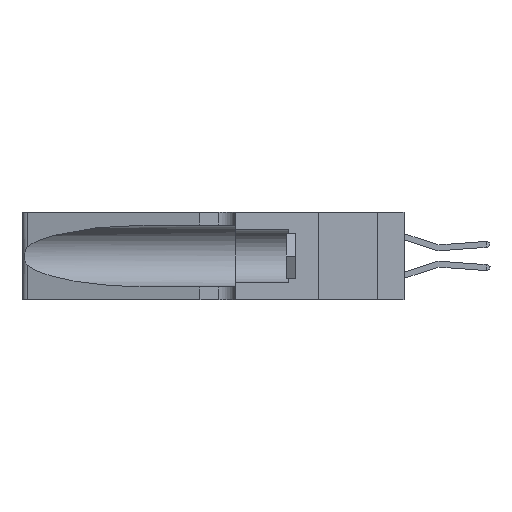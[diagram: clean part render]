
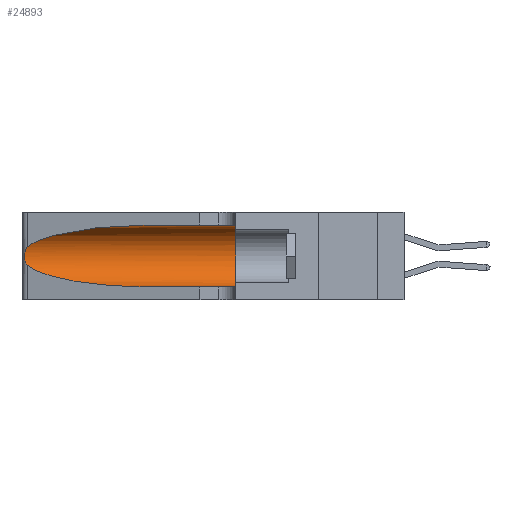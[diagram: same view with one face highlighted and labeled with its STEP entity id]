
A CAD part, left-side view. The second image highlights one B-rep face of the part: STEP entity #24893.
In plain terms, the highlighted cylindrical face has radius 3.308 mm (diameter 6.617 mm), a partial arc.
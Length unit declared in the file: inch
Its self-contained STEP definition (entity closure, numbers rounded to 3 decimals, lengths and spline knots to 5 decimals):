
#464 = CARTESIAN_POINT ( 'NONE',  ( 0.1305, 1.61858, 0.31525 ) ) ;
#783 = CIRCLE ( 'NONE', #27020, 0.13025 ) ;
#978 = CARTESIAN_POINT ( 'NONE',  ( 0.1305, 0.72297, 0.31525 ) ) ;
#1686 = CARTESIAN_POINT ( 'NONE',  ( 0.25487, 1.22718, 0.14631 ) ) ;
#2050 = EDGE_CURVE ( 'NONE', #2422, #31044, #10389, .T. ) ;
#2157 = DIRECTION ( 'NONE',  ( 0., -1., 0. ) ) ;
#2422 = VERTEX_POINT ( 'NONE', #22858 ) ;
#2440 = CARTESIAN_POINT ( 'NONE',  ( 0.1305, 0.35, 0.05475 ) ) ;
#3281 =( BOUNDED_CURVE ( )  B_SPLINE_CURVE ( 3, ( #1686, #19780, #32725, #7276 ),
 .UNSPECIFIED., .F., .F. ) 
 B_SPLINE_CURVE_WITH_KNOTS ( ( 4, 4 ),
 ( 3.44316, 4.71239 ),
 .UNSPECIFIED. ) 
 CURVE ( )  GEOMETRIC_REPRESENTATION_ITEM ( )  RATIONAL_B_SPLINE_CURVE ( ( 1., 0.87, 0.87, 1. ) ) 
 REPRESENTATION_ITEM ( '' )  );
#3384 = CARTESIAN_POINT ( 'NONE',  ( 0.18966, 0.96281, 0.31525 ) ) ;
#4279 = EDGE_CURVE ( 'NONE', #29355, #11122, #783, .T. ) ;
#4359 = VECTOR ( 'NONE', #30156, 39.37008 ) ;
#4670 = CARTESIAN_POINT ( 'NONE',  ( 0.26017, 1.23833, 0.17102 ) ) ;
#5508 = CARTESIAN_POINT ( 'NONE',  ( 0.25856, 1.23593, 0.16098 ) ) ;
#5982 = CARTESIAN_POINT ( 'NONE',  ( 0.2373, 1.15595, 0.28018 ) ) ;
#6266 = LINE ( 'NONE', #9989, #19621 ) ;
#6435 = CARTESIAN_POINT ( 'NONE',  ( 0.25787, 1.23484, 0.2124 ) ) ;
#6599 = ORIENTED_EDGE ( 'NONE', *, *, #18024, .T. ) ;
#7276 = CARTESIAN_POINT ( 'NONE',  ( 0.1305, 0.72297, 0.05475 ) ) ;
#9112 = CARTESIAN_POINT ( 'NONE',  ( 0.25555, 1.22993, 0.14849 ) ) ;
#9121 = EDGE_LOOP ( 'NONE', ( #25221, #6599, #23235, #28453, #20481, #32669 ) ) ;
#9911 = DIRECTION ( 'NONE',  ( 0., 1., 0. ) ) ;
#9989 = CARTESIAN_POINT ( 'NONE',  ( 0.1305, 1.61858, 0.05475 ) ) ;
#10095 = EDGE_CURVE ( 'NONE', #12147, #11122, #6266, .T. ) ;
#10389 =( BOUNDED_CURVE ( )  B_SPLINE_CURVE ( 3, ( #978, #3384, #5982, #32279 ),
 .UNSPECIFIED., .F., .F. ) 
 B_SPLINE_CURVE_WITH_KNOTS ( ( 4, 4 ),
 ( 1.5708, 2.84003 ),
 .UNSPECIFIED. ) 
 CURVE ( )  GEOMETRIC_REPRESENTATION_ITEM ( )  RATIONAL_B_SPLINE_CURVE ( ( 1., 0.87, 0.87, 1. ) ) 
 REPRESENTATION_ITEM ( '' )  );
#10783 = CARTESIAN_POINT ( 'NONE',  ( 0.25639, 1.23184, 0.21858 ) ) ;
#11122 = VERTEX_POINT ( 'NONE', #2440 ) ;
#11601 = CARTESIAN_POINT ( 'NONE',  ( 0.25639, 1.23186, 0.15144 ) ) ;
#12147 = VERTEX_POINT ( 'NONE', #30182 ) ;
#12367 = CYLINDRICAL_SURFACE ( 'NONE', #30223, 0.13025 ) ;
#12878 = LINE ( 'NONE', #464, #4359 ) ;
#14445 = EDGE_CURVE ( 'NONE', #33296, #12147, #3281, .T. ) ;
#14661 = CARTESIAN_POINT ( 'NONE',  ( 0.25487, 1.22718, 0.14631 ) ) ;
#15107 = DIRECTION ( 'NONE',  ( 0., 0., 1. ) ) ;
#15167 = CARTESIAN_POINT ( 'NONE',  ( 0.1305, 1.61858, 0.185 ) ) ;
#15740 = B_SPLINE_CURVE_WITH_KNOTS ( 'NONE', 3,
 ( #20543, #30998, #10783, #6435, #27950, #22853, #28835, #26338, #4670, #5508, #29528, #11601, #9112, #27048 ),
 .UNSPECIFIED., .F., .F.,
 ( 4, 2, 2, 2, 2, 2, 4 ),
 ( 0., 0.00027, 0.00053, 0.00107, 0.0016, 0.00187, 0.00214 ),
 .UNSPECIFIED. ) ;
#16672 = CARTESIAN_POINT ( 'NONE',  ( 0.1305, 0.35, 0.31525 ) ) ;
#17862 = CARTESIAN_POINT ( 'NONE',  ( 0.25487, 1.22718, 0.22369 ) ) ;
#18024 = EDGE_CURVE ( 'NONE', #31044, #33296, #15740, .T. ) ;
#19621 = VECTOR ( 'NONE', #32845, 39.37008 ) ;
#19780 = CARTESIAN_POINT ( 'NONE',  ( 0.2373, 1.15595, 0.08982 ) ) ;
#20481 = ORIENTED_EDGE ( 'NONE', *, *, #4279, .F. ) ;
#20543 = CARTESIAN_POINT ( 'NONE',  ( 0.25487, 1.22718, 0.22369 ) ) ;
#22853 = CARTESIAN_POINT ( 'NONE',  ( 0.26018, 1.23835, 0.19895 ) ) ;
#22858 = CARTESIAN_POINT ( 'NONE',  ( 0.1305, 0.72297, 0.31525 ) ) ;
#23235 = ORIENTED_EDGE ( 'NONE', *, *, #14445, .T. ) ;
#23599 = EDGE_CURVE ( 'NONE', #2422, #29355, #12878, .T. ) ;
#24893 = ADVANCED_FACE ( 'NONE', ( #25685 ), #12367, .F. ) ;
#25221 = ORIENTED_EDGE ( 'NONE', *, *, #2050, .T. ) ;
#25685 = FACE_OUTER_BOUND ( 'NONE', #9121, .T. ) ;
#25761 = CARTESIAN_POINT ( 'NONE',  ( 0.1305, 0.35, 0.185 ) ) ;
#26338 = CARTESIAN_POINT ( 'NONE',  ( 0.26075, 1.23896, 0.178 ) ) ;
#27020 = AXIS2_PLACEMENT_3D ( 'NONE', #25761, #9911, #15107 ) ;
#27048 = CARTESIAN_POINT ( 'NONE',  ( 0.25487, 1.22718, 0.14631 ) ) ;
#27777 = DIRECTION ( 'NONE',  ( 0., 0., -1. ) ) ;
#27950 = CARTESIAN_POINT ( 'NONE',  ( 0.25854, 1.2359, 0.20912 ) ) ;
#28453 = ORIENTED_EDGE ( 'NONE', *, *, #10095, .T. ) ;
#28835 = CARTESIAN_POINT ( 'NONE',  ( 0.26075, 1.23896, 0.19203 ) ) ;
#29355 = VERTEX_POINT ( 'NONE', #16672 ) ;
#29528 = CARTESIAN_POINT ( 'NONE',  ( 0.25789, 1.23486, 0.15765 ) ) ;
#30156 = DIRECTION ( 'NONE',  ( 0., -1., 0. ) ) ;
#30182 = CARTESIAN_POINT ( 'NONE',  ( 0.1305, 0.72297, 0.05475 ) ) ;
#30223 = AXIS2_PLACEMENT_3D ( 'NONE', #15167, #2157, #27777 ) ;
#30998 = CARTESIAN_POINT ( 'NONE',  ( 0.25555, 1.22994, 0.2215 ) ) ;
#31044 = VERTEX_POINT ( 'NONE', #17862 ) ;
#32279 = CARTESIAN_POINT ( 'NONE',  ( 0.25487, 1.22718, 0.22369 ) ) ;
#32669 = ORIENTED_EDGE ( 'NONE', *, *, #23599, .F. ) ;
#32725 = CARTESIAN_POINT ( 'NONE',  ( 0.18966, 0.96281, 0.05475 ) ) ;
#32845 = DIRECTION ( 'NONE',  ( 0., -1., 0. ) ) ;
#33296 = VERTEX_POINT ( 'NONE', #14661 ) ;
